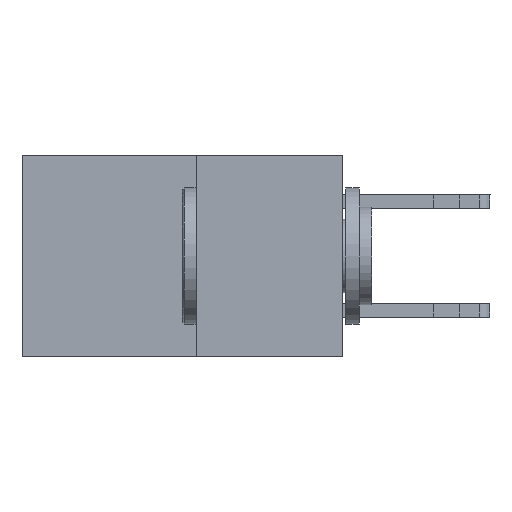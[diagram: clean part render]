
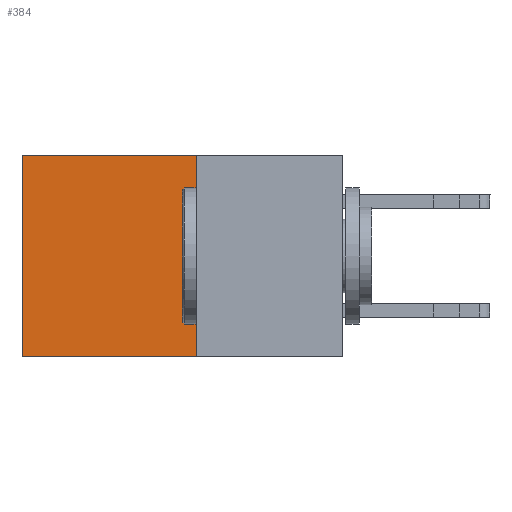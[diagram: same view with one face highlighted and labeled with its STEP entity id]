
A CAD part, left-side view. The second image highlights one B-rep face of the part: STEP entity #384.
In plain terms, the highlighted planar face has unit normal (-1, 0, 0).
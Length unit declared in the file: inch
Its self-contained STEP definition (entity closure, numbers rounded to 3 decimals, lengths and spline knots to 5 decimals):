
#71 = VERTEX_POINT ( 'NONE', #618 ) ;
#191 = VERTEX_POINT ( 'NONE', #1183 ) ;
#384 = ADVANCED_FACE ( 'NONE', ( #10232 ), #1324, .F. ) ;
#417 = VERTEX_POINT ( 'NONE', #5359 ) ;
#618 = CARTESIAN_POINT ( 'NONE',  ( 0.277, 0.59, 0. ) ) ;
#726 = ORIENTED_EDGE ( 'NONE', *, *, #8976, .F. ) ;
#1077 = LINE ( 'NONE', #13149, #5902 ) ;
#1183 = CARTESIAN_POINT ( 'NONE',  ( 0.277, 0.59, -0.37 ) ) ;
#1194 = EDGE_CURVE ( 'NONE', #71, #191, #1077, .T. ) ;
#1324 = PLANE ( 'NONE',  #3477 ) ;
#1773 = LINE ( 'NONE', #9392, #1843 ) ;
#1843 = VECTOR ( 'NONE', #5969, 39.37008 ) ;
#1993 = EDGE_CURVE ( 'NONE', #417, #191, #1773, .T. ) ;
#2204 = ORIENTED_EDGE ( 'NONE', *, *, #10003, .T. ) ;
#3179 = CARTESIAN_POINT ( 'NONE',  ( 0.277, 0.27, -0.37 ) ) ;
#3477 = AXIS2_PLACEMENT_3D ( 'NONE', #5672, #10024, #8946 ) ;
#3809 = VERTEX_POINT ( 'NONE', #8056 ) ;
#4110 = ORIENTED_EDGE ( 'NONE', *, *, #1993, .F. ) ;
#4551 = LINE ( 'NONE', #12279, #12720 ) ;
#5359 = CARTESIAN_POINT ( 'NONE',  ( 0.277, 0.27, -0.37 ) ) ;
#5672 = CARTESIAN_POINT ( 'NONE',  ( 0.277, 0.27, -0.37 ) ) ;
#5902 = VECTOR ( 'NONE', #6486, 39.37008 ) ;
#5969 = DIRECTION ( 'NONE',  ( 0., 1., 0. ) ) ;
#6486 = DIRECTION ( 'NONE',  ( 0., 0., -1. ) ) ;
#7584 = ORIENTED_EDGE ( 'NONE', *, *, #1194, .T. ) ;
#8056 = CARTESIAN_POINT ( 'NONE',  ( 0.277, 0.27, 0. ) ) ;
#8946 = DIRECTION ( 'NONE',  ( 0., 0., -1. ) ) ;
#8976 = EDGE_CURVE ( 'NONE', #3809, #417, #9538, .T. ) ;
#9392 = CARTESIAN_POINT ( 'NONE',  ( 0.277, 0.27, -0.37 ) ) ;
#9538 = LINE ( 'NONE', #3179, #12209 ) ;
#10003 = EDGE_CURVE ( 'NONE', #3809, #71, #4551, .T. ) ;
#10024 = DIRECTION ( 'NONE',  ( 1., 0., 0. ) ) ;
#10061 = EDGE_LOOP ( 'NONE', ( #7584, #4110, #726, #2204 ) ) ;
#10232 = FACE_OUTER_BOUND ( 'NONE', #10061, .T. ) ;
#11915 = DIRECTION ( 'NONE',  ( 0., 0., -1. ) ) ;
#12209 = VECTOR ( 'NONE', #11915, 39.37008 ) ;
#12279 = CARTESIAN_POINT ( 'NONE',  ( 0.277, 0.27, 0. ) ) ;
#12720 = VECTOR ( 'NONE', #13147, 39.37008 ) ;
#13147 = DIRECTION ( 'NONE',  ( 0., 1., 0. ) ) ;
#13149 = CARTESIAN_POINT ( 'NONE',  ( 0.277, 0.59, -0.37 ) ) ;
